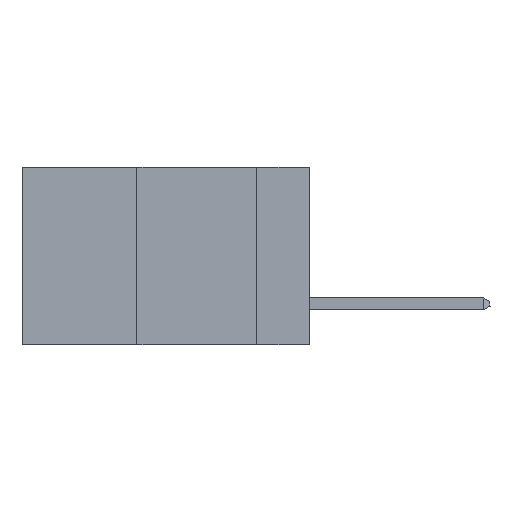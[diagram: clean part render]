
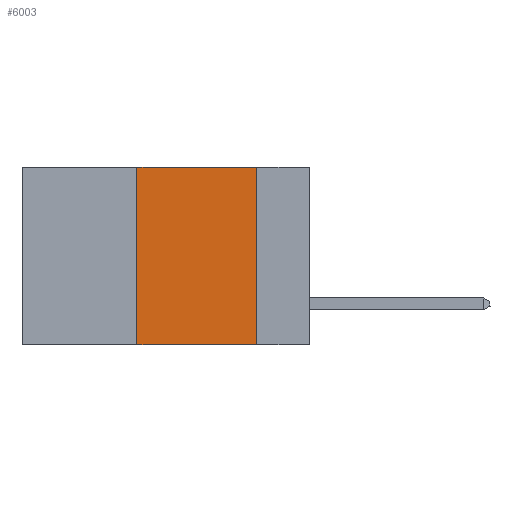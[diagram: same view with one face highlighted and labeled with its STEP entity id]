
A CAD part, left-side view. The second image highlights one B-rep face of the part: STEP entity #6003.
In plain terms, the highlighted planar face has unit normal (-1, 0, 0).
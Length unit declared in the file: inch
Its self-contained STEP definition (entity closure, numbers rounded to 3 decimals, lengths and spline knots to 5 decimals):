
#241 = DIRECTION ( 'NONE',  ( 0., 0., 1. ) ) ;
#618 = VERTEX_POINT ( 'NONE', #7414 ) ;
#640 = PLANE ( 'NONE',  #1356 ) ;
#1004 = VECTOR ( 'NONE', #241, 39.37008 ) ;
#1356 = AXIS2_PLACEMENT_3D ( 'NONE', #4302, #12886, #10221 ) ;
#1516 = CARTESIAN_POINT ( 'NONE',  ( 0., 0.36, -0.37 ) ) ;
#1662 = DIRECTION ( 'NONE',  ( 0., 0., -1. ) ) ;
#2424 = VERTEX_POINT ( 'NONE', #1516 ) ;
#3055 = ORIENTED_EDGE ( 'NONE', *, *, #7923, .T. ) ;
#3067 = VECTOR ( 'NONE', #8862, 39.37008 ) ;
#3245 = LINE ( 'NONE', #5127, #1004 ) ;
#3645 = ORIENTED_EDGE ( 'NONE', *, *, #13189, .F. ) ;
#4158 = ORIENTED_EDGE ( 'NONE', *, *, #8383, .F. ) ;
#4302 = CARTESIAN_POINT ( 'NONE',  ( 0., 0.6, 0. ) ) ;
#4437 = CARTESIAN_POINT ( 'NONE',  ( 0., 0.6, -0.37 ) ) ;
#5127 = CARTESIAN_POINT ( 'NONE',  ( 0., 0.36, 0. ) ) ;
#5225 = CARTESIAN_POINT ( 'NONE',  ( 0., 0.11, 0. ) ) ;
#6003 = ADVANCED_FACE ( 'NONE', ( #13431 ), #640, .F. ) ;
#6331 = CARTESIAN_POINT ( 'NONE',  ( 0., 0.6, 0. ) ) ;
#7414 = CARTESIAN_POINT ( 'NONE',  ( 0., 0.36, 0. ) ) ;
#7475 = LINE ( 'NONE', #6331, #3067 ) ;
#7691 = EDGE_LOOP ( 'NONE', ( #9598, #4158, #3645, #3055 ) ) ;
#7923 = EDGE_CURVE ( 'NONE', #2424, #9945, #9918, .T. ) ;
#8383 = EDGE_CURVE ( 'NONE', #618, #8785, #7475, .T. ) ;
#8433 = EDGE_CURVE ( 'NONE', #8785, #9945, #8957, .T. ) ;
#8785 = VERTEX_POINT ( 'NONE', #13559 ) ;
#8862 = DIRECTION ( 'NONE',  ( 0., -1., 0. ) ) ;
#8957 = LINE ( 'NONE', #5225, #15036 ) ;
#9598 = ORIENTED_EDGE ( 'NONE', *, *, #8433, .F. ) ;
#9918 = LINE ( 'NONE', #4437, #15045 ) ;
#9945 = VERTEX_POINT ( 'NONE', #11147 ) ;
#10221 = DIRECTION ( 'NONE',  ( 0., 0., -1. ) ) ;
#11147 = CARTESIAN_POINT ( 'NONE',  ( 0., 0.11, -0.37 ) ) ;
#12886 = DIRECTION ( 'NONE',  ( 1., 0., 0. ) ) ;
#13189 = EDGE_CURVE ( 'NONE', #2424, #618, #3245, .T. ) ;
#13431 = FACE_OUTER_BOUND ( 'NONE', #7691, .T. ) ;
#13559 = CARTESIAN_POINT ( 'NONE',  ( 0., 0.11, 0. ) ) ;
#14352 = DIRECTION ( 'NONE',  ( 0., -1., 0. ) ) ;
#15036 = VECTOR ( 'NONE', #1662, 39.37008 ) ;
#15045 = VECTOR ( 'NONE', #14352, 39.37008 ) ;
